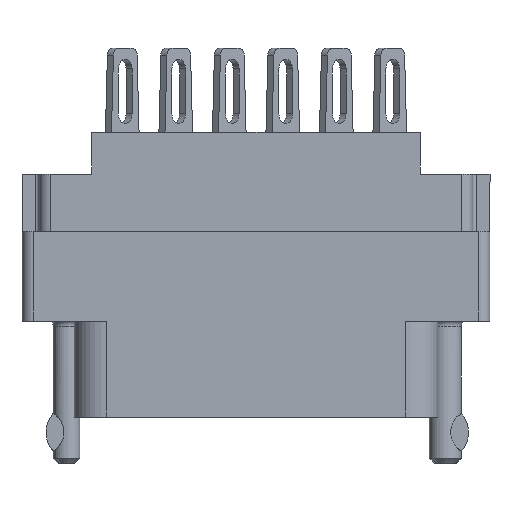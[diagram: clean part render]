
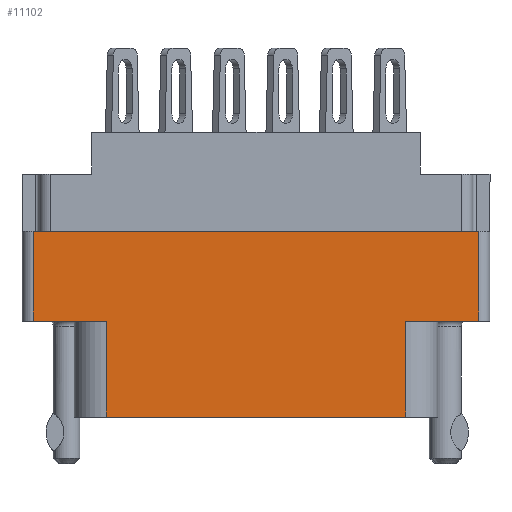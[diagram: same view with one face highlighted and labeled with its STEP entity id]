
A CAD part, front view. The second image highlights one B-rep face of the part: STEP entity #11102.
In plain terms, the highlighted planar face has unit normal (0, -1, 0).
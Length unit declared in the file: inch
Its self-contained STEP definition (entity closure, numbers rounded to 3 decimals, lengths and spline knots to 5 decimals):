
#380 = DIRECTION ( 'NONE',  ( 0., 0., -1. ) ) ;
#515 = EDGE_CURVE ( 'NONE', #11112, #9308, #4157, .T. ) ;
#1616 = CARTESIAN_POINT ( 'NONE',  ( 0.624, -0.343, -0.277 ) ) ;
#1739 = CARTESIAN_POINT ( 'NONE',  ( 0.624, -0.343, -0.798 ) ) ;
#2132 = CARTESIAN_POINT ( 'NONE',  ( 0.624, -0.343, -0.529 ) ) ;
#2373 = CARTESIAN_POINT ( 'NONE',  ( -0.624, -0.343, -0.277 ) ) ;
#2784 = VECTOR ( 'NONE', #30602, 39.37008 ) ;
#3888 = DIRECTION ( 'NONE',  ( 0., 0., 1. ) ) ;
#3890 = EDGE_CURVE ( 'NONE', #13529, #12466, #14977, .T. ) ;
#4157 = LINE ( 'NONE', #23534, #8252 ) ;
#4496 = VECTOR ( 'NONE', #380, 39.37008 ) ;
#5320 = VERTEX_POINT ( 'NONE', #29109 ) ;
#5578 = LINE ( 'NONE', #1739, #2784 ) ;
#5693 = ORIENTED_EDGE ( 'NONE', *, *, #6597, .F. ) ;
#6597 = EDGE_CURVE ( 'NONE', #13529, #11112, #22069, .T. ) ;
#7994 = EDGE_CURVE ( 'NONE', #28153, #5320, #16309, .T. ) ;
#8074 = CARTESIAN_POINT ( 'NONE',  ( 0.42, -0.343, -0.529 ) ) ;
#8252 = VECTOR ( 'NONE', #15714, 39.37008 ) ;
#8427 = DIRECTION ( 'NONE',  ( 0., 0., -1. ) ) ;
#8764 = VECTOR ( 'NONE', #8427, 39.37008 ) ;
#9221 = ORIENTED_EDGE ( 'NONE', *, *, #515, .F. ) ;
#9238 = LINE ( 'NONE', #20643, #11301 ) ;
#9294 = CARTESIAN_POINT ( 'NONE',  ( -0.42, -0.343, -0.529 ) ) ;
#9308 = VERTEX_POINT ( 'NONE', #1616 ) ;
#10229 = VECTOR ( 'NONE', #21446, 39.37008 ) ;
#10316 = PLANE ( 'NONE',  #19429 ) ;
#10948 = CARTESIAN_POINT ( 'NONE',  ( -0.42, -0.343, -0.529 ) ) ;
#11102 = ADVANCED_FACE ( 'NONE', ( #15349 ), #10316, .T. ) ;
#11112 = VERTEX_POINT ( 'NONE', #2373 ) ;
#11144 = EDGE_CURVE ( 'NONE', #15197, #29720, #9238, .T. ) ;
#11301 = VECTOR ( 'NONE', #12926, 39.37008 ) ;
#12466 = VERTEX_POINT ( 'NONE', #9294 ) ;
#12926 = DIRECTION ( 'NONE',  ( -1., 0., 0. ) ) ;
#13074 = ORIENTED_EDGE ( 'NONE', *, *, #3890, .T. ) ;
#13505 = ORIENTED_EDGE ( 'NONE', *, *, #25545, .F. ) ;
#13529 = VERTEX_POINT ( 'NONE', #29958 ) ;
#13622 = ORIENTED_EDGE ( 'NONE', *, *, #11144, .F. ) ;
#14977 = LINE ( 'NONE', #33279, #20673 ) ;
#15197 = VERTEX_POINT ( 'NONE', #2132 ) ;
#15349 = FACE_OUTER_BOUND ( 'NONE', #15636, .T. ) ;
#15541 = DIRECTION ( 'NONE',  ( 0., 0., -1. ) ) ;
#15636 = EDGE_LOOP ( 'NONE', ( #19069, #30295, #13505, #13622, #29373, #9221, #5693, #13074 ) ) ;
#15714 = DIRECTION ( 'NONE',  ( 1., 0., 0. ) ) ;
#16309 = LINE ( 'NONE', #21558, #10229 ) ;
#17084 = CARTESIAN_POINT ( 'NONE',  ( -0.624, -0.343, -0.798 ) ) ;
#17931 = DIRECTION ( 'NONE',  ( 1., 0., 0. ) ) ;
#19069 = ORIENTED_EDGE ( 'NONE', *, *, #21963, .T. ) ;
#19429 = AXIS2_PLACEMENT_3D ( 'NONE', #31122, #23008, #15541 ) ;
#20643 = CARTESIAN_POINT ( 'NONE',  ( 0., -0.343, -0.529 ) ) ;
#20673 = VECTOR ( 'NONE', #17931, 39.37008 ) ;
#21446 = DIRECTION ( 'NONE',  ( 1., 0., 0. ) ) ;
#21558 = CARTESIAN_POINT ( 'NONE',  ( -0.624, -0.343, -0.798 ) ) ;
#21963 = EDGE_CURVE ( 'NONE', #12466, #28153, #25413, .T. ) ;
#22069 = LINE ( 'NONE', #17084, #28165 ) ;
#23008 = DIRECTION ( 'NONE',  ( 0., -1., 0. ) ) ;
#23534 = CARTESIAN_POINT ( 'NONE',  ( -0.656, -0.343, -0.277 ) ) ;
#25174 = CARTESIAN_POINT ( 'NONE',  ( -0.42, -0.343, -0.798 ) ) ;
#25413 = LINE ( 'NONE', #10948, #8764 ) ;
#25545 = EDGE_CURVE ( 'NONE', #29720, #5320, #27680, .T. ) ;
#27680 = LINE ( 'NONE', #8074, #4496 ) ;
#28153 = VERTEX_POINT ( 'NONE', #25174 ) ;
#28165 = VECTOR ( 'NONE', #3888, 39.37008 ) ;
#29109 = CARTESIAN_POINT ( 'NONE',  ( 0.42, -0.343, -0.798 ) ) ;
#29373 = ORIENTED_EDGE ( 'NONE', *, *, #33038, .T. ) ;
#29720 = VERTEX_POINT ( 'NONE', #33519 ) ;
#29958 = CARTESIAN_POINT ( 'NONE',  ( -0.624, -0.343, -0.529 ) ) ;
#30295 = ORIENTED_EDGE ( 'NONE', *, *, #7994, .T. ) ;
#30602 = DIRECTION ( 'NONE',  ( 0., 0., 1. ) ) ;
#31122 = CARTESIAN_POINT ( 'NONE',  ( -0.624, -0.343, -0.798 ) ) ;
#33038 = EDGE_CURVE ( 'NONE', #15197, #9308, #5578, .T. ) ;
#33279 = CARTESIAN_POINT ( 'NONE',  ( 0., -0.343, -0.529 ) ) ;
#33519 = CARTESIAN_POINT ( 'NONE',  ( 0.42, -0.343, -0.529 ) ) ;
